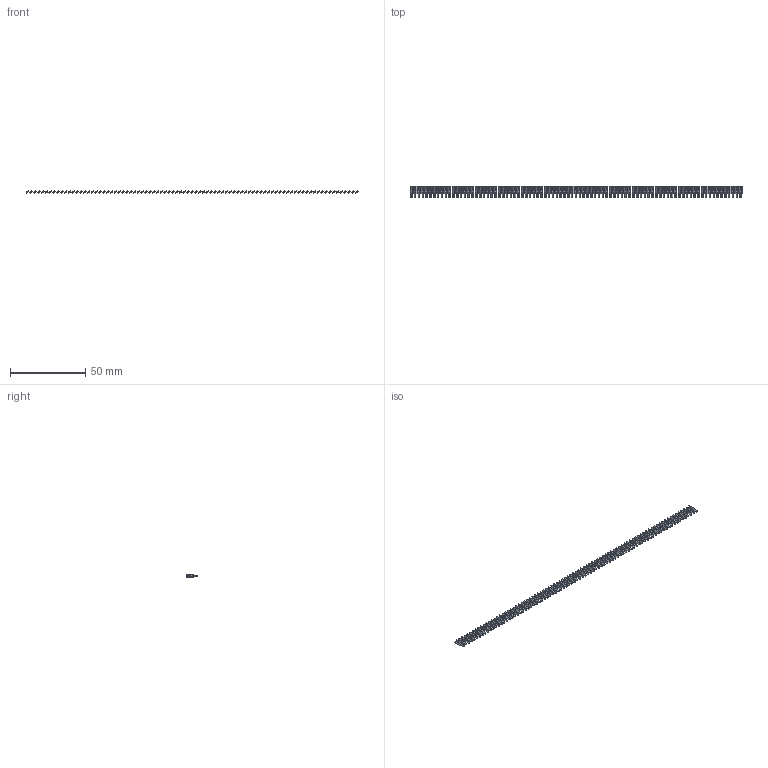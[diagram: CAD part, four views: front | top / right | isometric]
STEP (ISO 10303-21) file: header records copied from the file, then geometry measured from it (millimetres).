
FILE_DESCRIPTION (( 'STEP AP203' ), '1' );
FILE_NAME ('106-087-253-100.STEP', '2020-04-16T22:59:25', ( '' ), ( '' ), 'SwSTEP 2.0', 'SolidWorks 2016', '' );
FILE_SCHEMA (( 'CONFIG_CONTROL_DESIGN' ));
Length unit declared in the file: inch
Products named in the file (2): 100-290-001_100-290-253; 106-087-253-100
Assembly tree (87 placements, depth 2):
  106-087-253-100
    100-290-001_100-290-253  x87
Bounding box: 220.24 x 7.62 x 1.8 mm (x, y, z)
Volume: 480 mm3; surface area: 2993.4 mm2
Topology: 87 solids, 87 shells, 1740 faces, 4698 edges, 3132 vertices
Faces by surface type: plane 1653, cylinder 87
Entity records: 3572 total; most frequent: DIRECTION 276, CARTESIAN_POINT 200, LOCAL_TIME 184, DATE_AND_TIME 184, CALENDAR_DATE 184, COORDINATED_UNIVERSAL_TIME_OFFSET 184, AXIS2_PLACEMENT_3D 112, ORIENTED_EDGE 108
